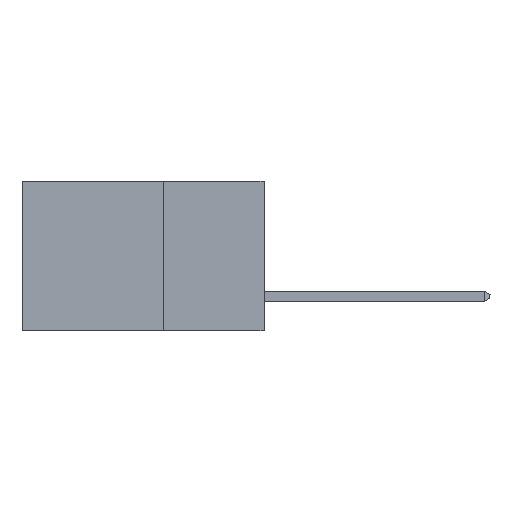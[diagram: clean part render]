
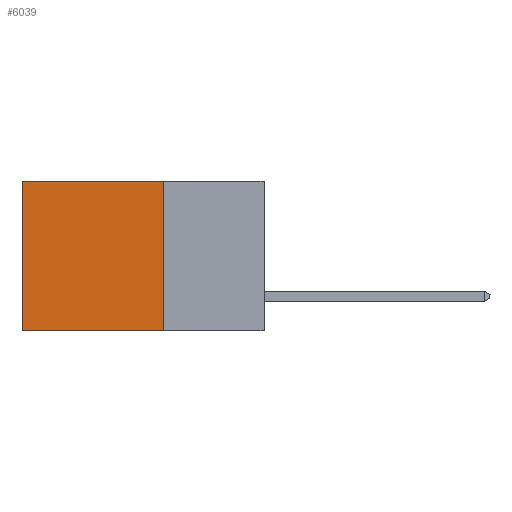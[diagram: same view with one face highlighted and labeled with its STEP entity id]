
A CAD part, left-side view. The second image highlights one B-rep face of the part: STEP entity #6039.
In plain terms, the highlighted planar face has unit normal (-1, 0, 0).
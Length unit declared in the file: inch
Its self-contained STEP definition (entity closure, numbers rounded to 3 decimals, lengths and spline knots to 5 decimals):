
#8 = CARTESIAN_POINT ( 'NONE',  ( 0.2615, 0.25, 0. ) ) ;
#369 = LINE ( 'NONE', #7914, #8421 ) ;
#718 = DIRECTION ( 'NONE',  ( 0., 0., -1. ) ) ;
#1054 = VERTEX_POINT ( 'NONE', #8 ) ;
#1151 = VERTEX_POINT ( 'NONE', #11504 ) ;
#1336 = EDGE_CURVE ( 'NONE', #1151, #11149, #369, .T. ) ;
#2009 = AXIS2_PLACEMENT_3D ( 'NONE', #10783, #6024, #6219 ) ;
#2341 = DIRECTION ( 'NONE',  ( 0., 1., 0. ) ) ;
#3298 = FACE_OUTER_BOUND ( 'NONE', #8036, .T. ) ;
#3422 = VECTOR ( 'NONE', #3955, 39.37008 ) ;
#3955 = DIRECTION ( 'NONE',  ( 0., 0., -1. ) ) ;
#4022 = ORIENTED_EDGE ( 'NONE', *, *, #6282, .T. ) ;
#5016 = LINE ( 'NONE', #10628, #3422 ) ;
#5237 = DIRECTION ( 'NONE',  ( 0., 1., 0. ) ) ;
#5423 = LINE ( 'NONE', #9186, #5893 ) ;
#5855 = LINE ( 'NONE', #9622, #11625 ) ;
#5893 = VECTOR ( 'NONE', #718, 39.37008 ) ;
#6024 = DIRECTION ( 'NONE',  ( 1., 0., 0. ) ) ;
#6039 = ADVANCED_FACE ( 'NONE', ( #3298 ), #11826, .F. ) ;
#6219 = DIRECTION ( 'NONE',  ( 0., 0., -1. ) ) ;
#6282 = EDGE_CURVE ( 'NONE', #9139, #11149, #5016, .T. ) ;
#6848 = CARTESIAN_POINT ( 'NONE',  ( 0.2615, 0.6, -0.37 ) ) ;
#7914 = CARTESIAN_POINT ( 'NONE',  ( 0.2615, 0.25, -0.37 ) ) ;
#8036 = EDGE_LOOP ( 'NONE', ( #4022, #8284, #11922, #11906 ) ) ;
#8260 = CARTESIAN_POINT ( 'NONE',  ( 0.2615, 0.6, 0. ) ) ;
#8284 = ORIENTED_EDGE ( 'NONE', *, *, #1336, .F. ) ;
#8421 = VECTOR ( 'NONE', #2341, 39.37008 ) ;
#9139 = VERTEX_POINT ( 'NONE', #8260 ) ;
#9186 = CARTESIAN_POINT ( 'NONE',  ( 0.2615, 0.25, -0.37 ) ) ;
#9225 = EDGE_CURVE ( 'NONE', #1054, #1151, #5423, .T. ) ;
#9622 = CARTESIAN_POINT ( 'NONE',  ( 0.2615, 0.25, 0. ) ) ;
#10241 = EDGE_CURVE ( 'NONE', #1054, #9139, #5855, .T. ) ;
#10628 = CARTESIAN_POINT ( 'NONE',  ( 0.2615, 0.6, -0.37 ) ) ;
#10783 = CARTESIAN_POINT ( 'NONE',  ( 0.2615, 0.25, -0.37 ) ) ;
#11149 = VERTEX_POINT ( 'NONE', #6848 ) ;
#11504 = CARTESIAN_POINT ( 'NONE',  ( 0.2615, 0.25, -0.37 ) ) ;
#11625 = VECTOR ( 'NONE', #5237, 39.37008 ) ;
#11826 = PLANE ( 'NONE',  #2009 ) ;
#11906 = ORIENTED_EDGE ( 'NONE', *, *, #10241, .T. ) ;
#11922 = ORIENTED_EDGE ( 'NONE', *, *, #9225, .F. ) ;
